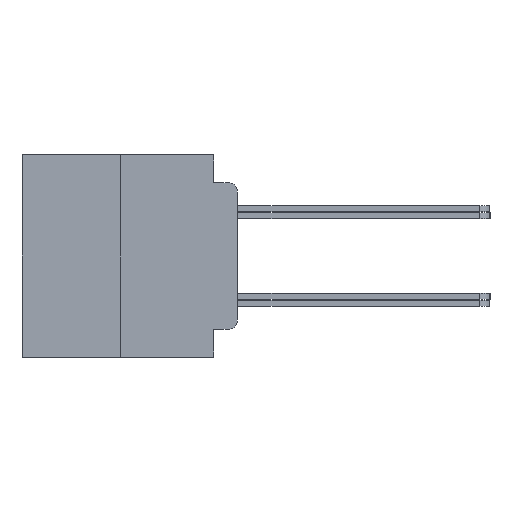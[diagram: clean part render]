
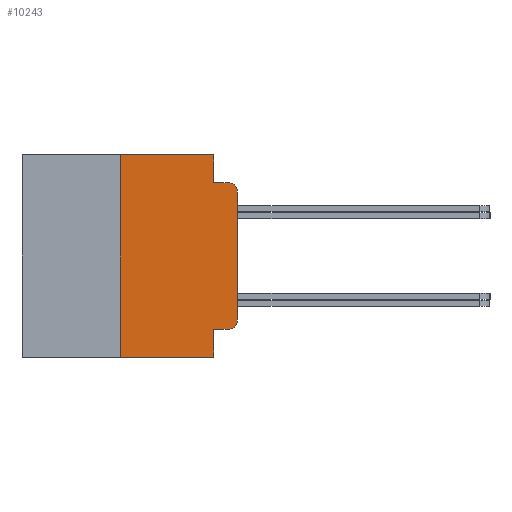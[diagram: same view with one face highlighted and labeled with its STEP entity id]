
A CAD part, left-side view. The second image highlights one B-rep face of the part: STEP entity #10243.
In plain terms, the highlighted planar face has unit normal (-1, 0, 0).
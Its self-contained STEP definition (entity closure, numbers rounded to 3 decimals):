
#175 = CARTESIAN_POINT ( 'NONE',  ( -75.603, 0.508, 3.467 ) ) ;
#382 = CARTESIAN_POINT ( 'NONE',  ( -75.603, 0., -3.467 ) ) ;
#509 = VECTOR ( 'NONE', #27800, 1000. ) ;
#643 = CIRCLE ( 'NONE', #8999, 0.508 ) ;
#721 = CARTESIAN_POINT ( 'NONE',  ( -75.603, 11.684, -5.486 ) ) ;
#767 = VERTEX_POINT ( 'NONE', #15373 ) ;
#1952 = CARTESIAN_POINT ( 'NONE',  ( -75.603, 0.508, 3.975 ) ) ;
#2482 = CARTESIAN_POINT ( 'NONE',  ( -75.603, 6.35, 5.486 ) ) ;
#3238 = VERTEX_POINT ( 'NONE', #2482 ) ;
#3367 = LINE ( 'NONE', #5028, #509 ) ;
#4534 = VERTEX_POINT ( 'NONE', #21457 ) ;
#4699 = ORIENTED_EDGE ( 'NONE', *, *, #7965, .F. ) ;
#4761 = AXIS2_PLACEMENT_3D ( 'NONE', #25889, #7598, #25779 ) ;
#4827 = VECTOR ( 'NONE', #18393, 1000. ) ;
#5028 = CARTESIAN_POINT ( 'NONE',  ( -75.603, 11.684, 5.486 ) ) ;
#5148 = DIRECTION ( 'NONE',  ( 0., -1., 0. ) ) ;
#5461 = VERTEX_POINT ( 'NONE', #7251 ) ;
#5902 = VECTOR ( 'NONE', #12786, 1000. ) ;
#6238 = LINE ( 'NONE', #7509, #22761 ) ;
#6750 = CARTESIAN_POINT ( 'NONE',  ( -75.603, 1.295, -3.975 ) ) ;
#6814 = VERTEX_POINT ( 'NONE', #1952 ) ;
#7038 = LINE ( 'NONE', #14559, #18555 ) ;
#7251 = CARTESIAN_POINT ( 'NONE',  ( -75.603, 1.295, 3.975 ) ) ;
#7509 = CARTESIAN_POINT ( 'NONE',  ( -75.603, 1.295, 0. ) ) ;
#7598 = DIRECTION ( 'NONE',  ( -1., 0., 0. ) ) ;
#7965 = EDGE_CURVE ( 'NONE', #767, #3238, #13123, .T. ) ;
#8002 = EDGE_CURVE ( 'NONE', #9902, #4534, #15299, .T. ) ;
#8999 = AXIS2_PLACEMENT_3D ( 'NONE', #175, #16576, #21049 ) ;
#9160 = VECTOR ( 'NONE', #13475, 1000. ) ;
#9902 = VERTEX_POINT ( 'NONE', #382 ) ;
#10243 = ADVANCED_FACE ( 'NONE', ( #19105 ), #17273, .F. ) ;
#10912 = ORIENTED_EDGE ( 'NONE', *, *, #11903, .T. ) ;
#11903 = EDGE_CURVE ( 'NONE', #4534, #6814, #643, .T. ) ;
#12061 = DIRECTION ( 'NONE',  ( 0., 0., -1. ) ) ;
#12328 = AXIS2_PLACEMENT_3D ( 'NONE', #26471, #17372, #19651 ) ;
#12786 = DIRECTION ( 'NONE',  ( 0., -1., 0. ) ) ;
#13123 = LINE ( 'NONE', #13274, #9160 ) ;
#13194 = VERTEX_POINT ( 'NONE', #13323 ) ;
#13274 = CARTESIAN_POINT ( 'NONE',  ( -75.603, 6.35, -5.486 ) ) ;
#13323 = CARTESIAN_POINT ( 'NONE',  ( -75.603, 1.295, 5.486 ) ) ;
#13475 = DIRECTION ( 'NONE',  ( 0., 0., 1. ) ) ;
#13742 = VECTOR ( 'NONE', #5148, 1000. ) ;
#14174 = CARTESIAN_POINT ( 'NONE',  ( -75.603, 1.295, -3.975 ) ) ;
#14559 = CARTESIAN_POINT ( 'NONE',  ( -75.603, 1.295, 0. ) ) ;
#14964 = CARTESIAN_POINT ( 'NONE',  ( -75.603, 1.295, -5.486 ) ) ;
#15299 = LINE ( 'NONE', #22312, #4827 ) ;
#15373 = CARTESIAN_POINT ( 'NONE',  ( -75.603, 6.35, -5.486 ) ) ;
#15441 = EDGE_CURVE ( 'NONE', #13194, #5461, #7038, .T. ) ;
#16319 = ORIENTED_EDGE ( 'NONE', *, *, #25160, .F. ) ;
#16576 = DIRECTION ( 'NONE',  ( -1., 0., 0. ) ) ;
#16651 = LINE ( 'NONE', #721, #13742 ) ;
#17273 = PLANE ( 'NONE',  #12328 ) ;
#17372 = DIRECTION ( 'NONE',  ( 1., 0., 0. ) ) ;
#18393 = DIRECTION ( 'NONE',  ( 0., 0., 1. ) ) ;
#18395 = DIRECTION ( 'NONE',  ( 0., -1., 0. ) ) ;
#18555 = VECTOR ( 'NONE', #28407, 1000. ) ;
#19105 = FACE_OUTER_BOUND ( 'NONE', #20388, .T. ) ;
#19318 = ORIENTED_EDGE ( 'NONE', *, *, #25642, .F. ) ;
#19510 = EDGE_CURVE ( 'NONE', #21005, #9902, #29214, .T. ) ;
#19562 = LINE ( 'NONE', #24113, #5902 ) ;
#19651 = DIRECTION ( 'NONE',  ( 0., 0., -1. ) ) ;
#19783 = ORIENTED_EDGE ( 'NONE', *, *, #27989, .T. ) ;
#20019 = ORIENTED_EDGE ( 'NONE', *, *, #29469, .T. ) ;
#20388 = EDGE_LOOP ( 'NONE', ( #19783, #28340, #27823, #10912, #16319, #21366, #19318, #4699, #20019, #28723 ) ) ;
#21005 = VERTEX_POINT ( 'NONE', #24857 ) ;
#21049 = DIRECTION ( 'NONE',  ( 0., 0., -1. ) ) ;
#21085 = VERTEX_POINT ( 'NONE', #6750 ) ;
#21366 = ORIENTED_EDGE ( 'NONE', *, *, #15441, .F. ) ;
#21457 = CARTESIAN_POINT ( 'NONE',  ( -75.603, 0., 3.467 ) ) ;
#22312 = CARTESIAN_POINT ( 'NONE',  ( -75.603, 0., 5.486 ) ) ;
#22761 = VECTOR ( 'NONE', #12061, 1000. ) ;
#24113 = CARTESIAN_POINT ( 'NONE',  ( -75.603, 1.295, 3.975 ) ) ;
#24857 = CARTESIAN_POINT ( 'NONE',  ( -75.603, 0.508, -3.975 ) ) ;
#24955 = VECTOR ( 'NONE', #18395, 1000. ) ;
#25160 = EDGE_CURVE ( 'NONE', #5461, #6814, #19562, .T. ) ;
#25606 = EDGE_CURVE ( 'NONE', #21085, #25872, #6238, .T. ) ;
#25642 = EDGE_CURVE ( 'NONE', #3238, #13194, #3367, .T. ) ;
#25779 = DIRECTION ( 'NONE',  ( 0., 0., -1. ) ) ;
#25872 = VERTEX_POINT ( 'NONE', #14964 ) ;
#25889 = CARTESIAN_POINT ( 'NONE',  ( -75.603, 0.508, -3.467 ) ) ;
#26471 = CARTESIAN_POINT ( 'NONE',  ( -75.603, 11.684, 5.486 ) ) ;
#27119 = LINE ( 'NONE', #14174, #24955 ) ;
#27800 = DIRECTION ( 'NONE',  ( 0., -1., 0. ) ) ;
#27823 = ORIENTED_EDGE ( 'NONE', *, *, #8002, .T. ) ;
#27989 = EDGE_CURVE ( 'NONE', #21085, #21005, #27119, .T. ) ;
#28340 = ORIENTED_EDGE ( 'NONE', *, *, #19510, .T. ) ;
#28407 = DIRECTION ( 'NONE',  ( 0., 0., -1. ) ) ;
#28723 = ORIENTED_EDGE ( 'NONE', *, *, #25606, .F. ) ;
#29214 = CIRCLE ( 'NONE', #4761, 0.508 ) ;
#29469 = EDGE_CURVE ( 'NONE', #767, #25872, #16651, .T. ) ;
